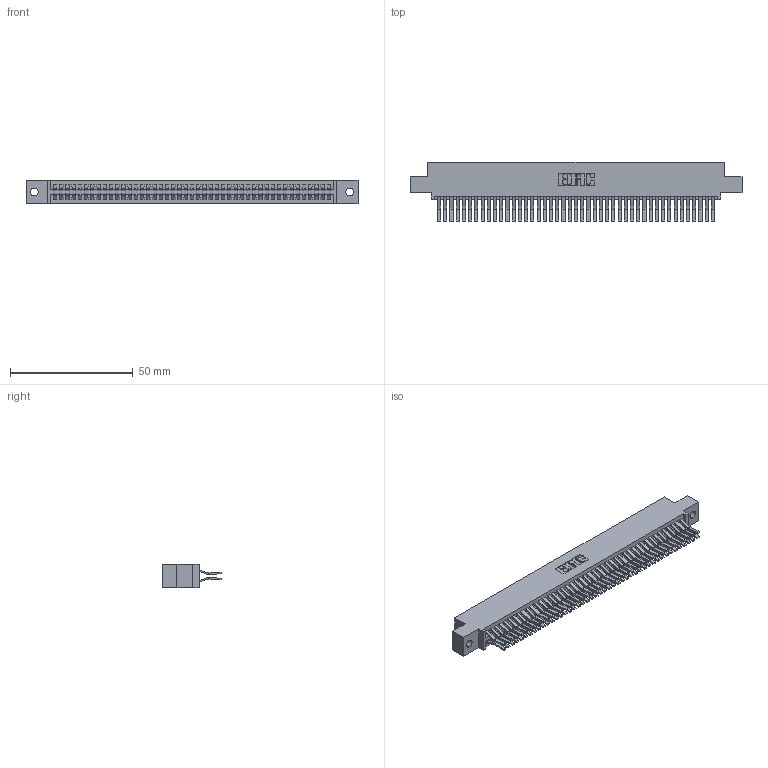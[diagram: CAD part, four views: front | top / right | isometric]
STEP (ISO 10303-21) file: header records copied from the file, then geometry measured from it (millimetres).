
FILE_DESCRIPTION (( 'STEP AP203' ), '1' );
FILE_NAME ('395-090-560-502.STEP', '2019-10-25T18:12:22', ( '' ), ( '' ), 'SwSTEP 2.0', 'SolidWorks 2016', '' );
FILE_SCHEMA (( 'CONFIG_CONTROL_DESIGN' ));
Length unit declared in the file: inch
Products named in the file (3): 345 Part_0.110 Offset - 0.128 Dia; 345-292-001_560 Tail; 395-090-560-502
Assembly tree (91 placements, depth 2):
  395-090-560-502
    345 Part_0.110 Offset - 0.128 Dia
    345-292-001_560 Tail  x90
Bounding box: 135.51 x 24.45 x 9.4 mm (x, y, z)
Volume: 13671.2 mm3; surface area: 21603.7 mm2
Topology: 91 solids, 91 shells, 4810 faces, 14303 edges, 9414 vertices
Faces by surface type: plane 3054, cylinder 1756
Entity records: 35127 total; most frequent: CARTESIAN_POINT 5888, ORIENTED_EDGE 5822, DIRECTION 5191, EDGE_CURVE 2911, LINE 2595, VECTOR 2595, VERTEX_POINT 1938, AXIS2_PLACEMENT_3D 1298
